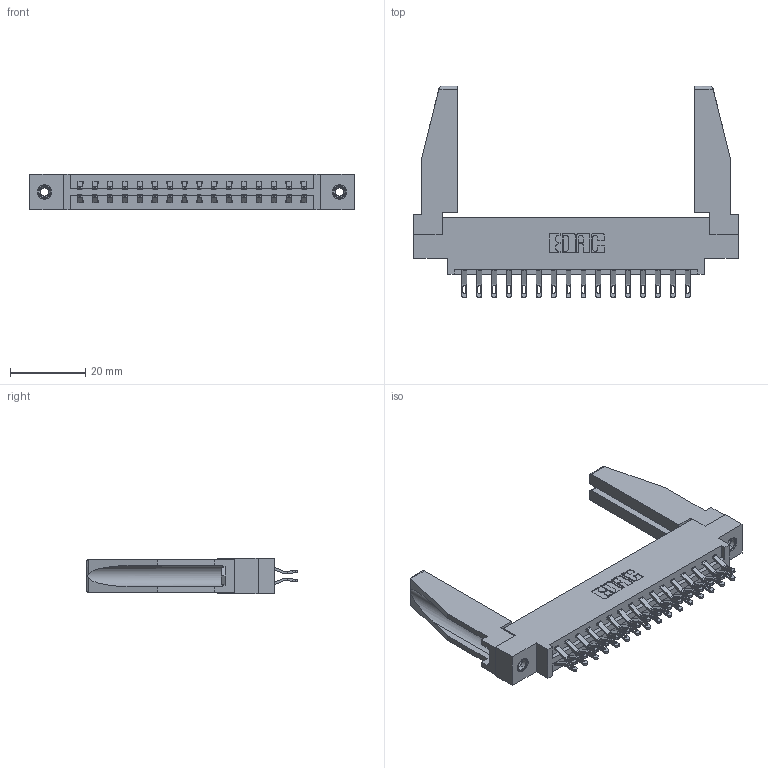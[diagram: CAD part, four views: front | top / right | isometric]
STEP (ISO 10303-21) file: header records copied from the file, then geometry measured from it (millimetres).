
FILE_DESCRIPTION (( 'STEP AP203' ), '1' );
FILE_NAME ('387-032-555-878.STEP', '2019-10-17T16:20:06', ( '' ), ( '' ), 'SwSTEP 2.0', 'SolidWorks 2016', '' );
FILE_SCHEMA (( 'CONFIG_CONTROL_DESIGN' ));
Length unit declared in the file: inch
Products named in the file (5): 345-292-001_555 Tail; 345-250-001_345-250-001-102; 387-032-555-878; 337 Part_0.170 Offset - 0.156 Dia-TI; 307-220-078
Assembly tree (37 placements, depth 2):
  387-032-555-878
    337 Part_0.170 Offset - 0.156 Dia-TI
    345-292-001_555 Tail  x32
    345-250-001_345-250-001-102  x2
    307-220-078  x2
Bounding box: 86.41 x 56.27 x 9.4 mm (x, y, z)
Volume: 12729.2 mm3; surface area: 13911.5 mm2
Topology: 37 solids, 37 shells, 2168 faces, 6701 edges, 4458 vertices
Faces by surface type: plane 1310, cylinder 842, cone 12, torus 4
Entity records: 18666 total; most frequent: CARTESIAN_POINT 3202, ORIENTED_EDGE 3064, DIRECTION 2748, EDGE_CURVE 1532, VECTOR 1346, LINE 1346, VERTEX_POINT 1016, AXIS2_PLACEMENT_3D 701
